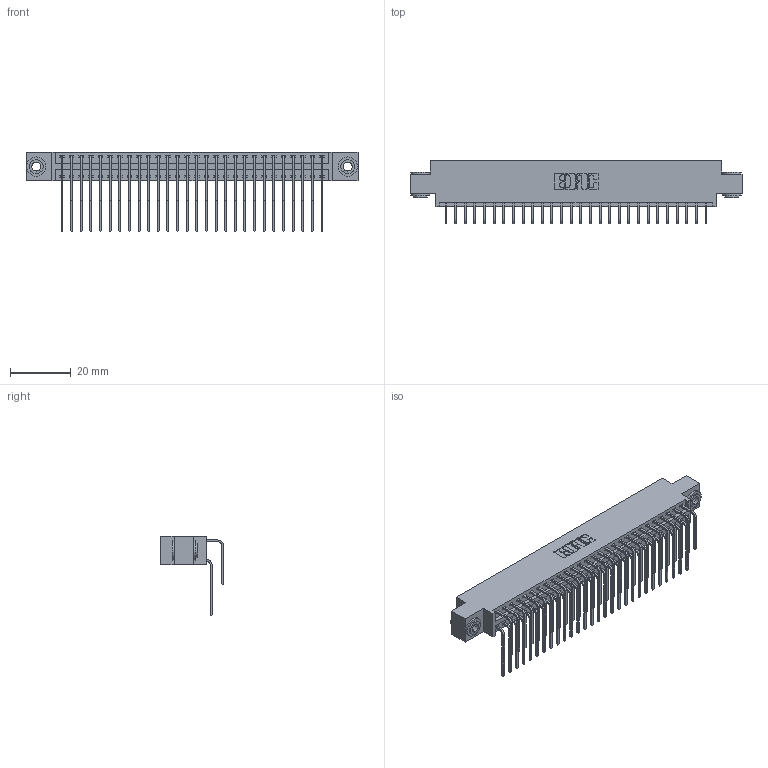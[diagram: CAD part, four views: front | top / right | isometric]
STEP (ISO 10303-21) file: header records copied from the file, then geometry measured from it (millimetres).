
FILE_DESCRIPTION (( 'STEP AP203' ), '1' );
FILE_NAME ('346-056-559-803.STEP', '2022-05-21T06:58:18', ( '' ), ( '' ), 'SwSTEP 2.0', 'SolidWorks 2020', '' );
FILE_SCHEMA (( 'CONFIG_CONTROL_DESIGN' ));
Length unit declared in the file: inch
Products named in the file (5): 345-292-001_558 559 Tail - 1; 345-292-001_559 Tail - 2; 346-056-559-803; 346 Part_0.170 Offset - 0.156 Dia-TH; 345-250-002_345-250-002-102
Assembly tree (59 placements, depth 2):
  346-056-559-803
    346 Part_0.170 Offset - 0.156 Dia-TH
    345-292-001_558 559 Tail - 1  x28
    345-292-001_559 Tail - 2  x28
    345-250-002_345-250-002-102  x2
Bounding box: 109.47 x 20.89 x 26.16 mm (x, y, z)
Volume: 10736.1 mm3; surface area: 16515.5 mm2
Topology: 59 solids, 59 shells, 3202 faces, 9469 edges, 6234 vertices
Faces by surface type: plane 2176, cylinder 1018, cone 8
Entity records: 23140 total; most frequent: CARTESIAN_POINT 3868, ORIENTED_EDGE 3742, DIRECTION 3461, EDGE_CURVE 1871, VECTOR 1563, LINE 1563, VERTEX_POINT 1242, AXIS2_PLACEMENT_3D 949
